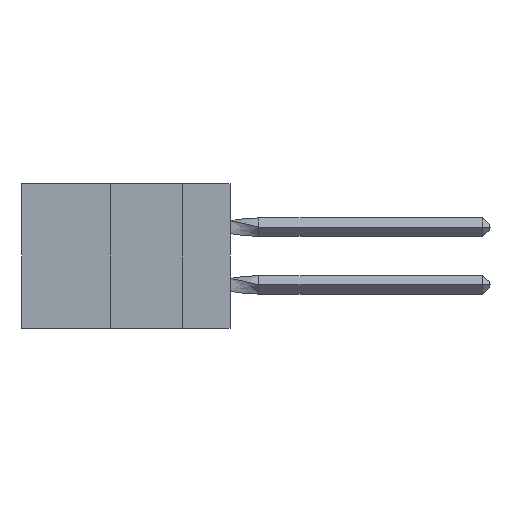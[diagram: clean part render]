
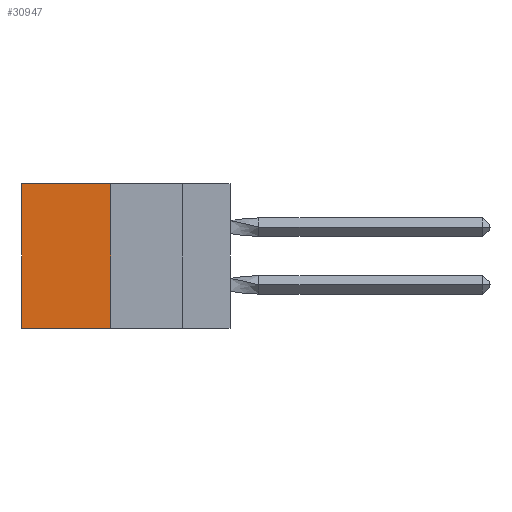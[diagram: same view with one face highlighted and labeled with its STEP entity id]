
A CAD part, left-side view. The second image highlights one B-rep face of the part: STEP entity #30947.
In plain terms, the highlighted planar face has unit normal (-1, 0, 0).
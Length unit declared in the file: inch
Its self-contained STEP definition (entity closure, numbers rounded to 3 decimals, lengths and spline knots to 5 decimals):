
#271 = CARTESIAN_POINT ( 'NONE',  ( 0.305, 0.413, -0.5 ) ) ;
#1849 = VERTEX_POINT ( 'NONE', #8758 ) ;
#1911 = CARTESIAN_POINT ( 'NONE',  ( 0.305, 0.72, -0.5 ) ) ;
#2126 = PLANE ( 'NONE',  #3881 ) ;
#3140 = EDGE_CURVE ( 'NONE', #33802, #34056, #11476, .T. ) ;
#3881 = AXIS2_PLACEMENT_3D ( 'NONE', #31605, #22475, #7577 ) ;
#6666 = DIRECTION ( 'NONE',  ( 0., 1., 0. ) ) ;
#6821 = EDGE_CURVE ( 'NONE', #1849, #36701, #25996, .T. ) ;
#7577 = DIRECTION ( 'NONE',  ( 0., 0., -1. ) ) ;
#8758 = CARTESIAN_POINT ( 'NONE',  ( 0.305, 0.413, -0.5 ) ) ;
#11476 = LINE ( 'NONE', #12504, #31483 ) ;
#12504 = CARTESIAN_POINT ( 'NONE',  ( 0.305, 0.413, 0. ) ) ;
#13011 = EDGE_LOOP ( 'NONE', ( #38108, #35173, #28090, #32861 ) ) ;
#14276 = FACE_OUTER_BOUND ( 'NONE', #13011, .T. ) ;
#15530 = CARTESIAN_POINT ( 'NONE',  ( 0.305, 0.72, 0. ) ) ;
#16557 = CARTESIAN_POINT ( 'NONE',  ( 0.305, 0.72, -0.5 ) ) ;
#17953 = DIRECTION ( 'NONE',  ( 0., 1., 0. ) ) ;
#22475 = DIRECTION ( 'NONE',  ( 1., 0., 0. ) ) ;
#25918 = CARTESIAN_POINT ( 'NONE',  ( 0.305, 0.413, 0. ) ) ;
#25959 = VECTOR ( 'NONE', #32354, 39.37008 ) ;
#25996 = LINE ( 'NONE', #29899, #33944 ) ;
#28090 = ORIENTED_EDGE ( 'NONE', *, *, #37448, .F. ) ;
#29899 = CARTESIAN_POINT ( 'NONE',  ( 0.305, 0.413, -0.5 ) ) ;
#30000 = VECTOR ( 'NONE', #31499, 39.37008 ) ;
#30947 = ADVANCED_FACE ( 'NONE', ( #14276 ), #2126, .F. ) ;
#31483 = VECTOR ( 'NONE', #6666, 39.37008 ) ;
#31499 = DIRECTION ( 'NONE',  ( 0., 0., -1. ) ) ;
#31605 = CARTESIAN_POINT ( 'NONE',  ( 0.305, 0.413, -0.5 ) ) ;
#32354 = DIRECTION ( 'NONE',  ( 0., 0., -1. ) ) ;
#32861 = ORIENTED_EDGE ( 'NONE', *, *, #3140, .T. ) ;
#33802 = VERTEX_POINT ( 'NONE', #25918 ) ;
#33944 = VECTOR ( 'NONE', #17953, 39.37008 ) ;
#34056 = VERTEX_POINT ( 'NONE', #15530 ) ;
#34282 = EDGE_CURVE ( 'NONE', #34056, #36701, #37919, .T. ) ;
#34813 = LINE ( 'NONE', #271, #25959 ) ;
#35173 = ORIENTED_EDGE ( 'NONE', *, *, #6821, .F. ) ;
#36701 = VERTEX_POINT ( 'NONE', #1911 ) ;
#37448 = EDGE_CURVE ( 'NONE', #33802, #1849, #34813, .T. ) ;
#37919 = LINE ( 'NONE', #16557, #30000 ) ;
#38108 = ORIENTED_EDGE ( 'NONE', *, *, #34282, .T. ) ;
